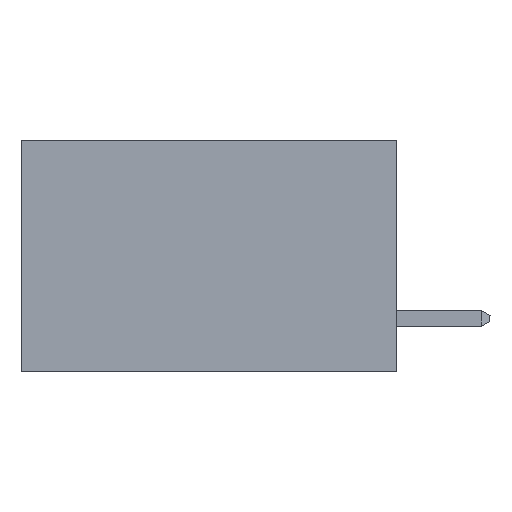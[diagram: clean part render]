
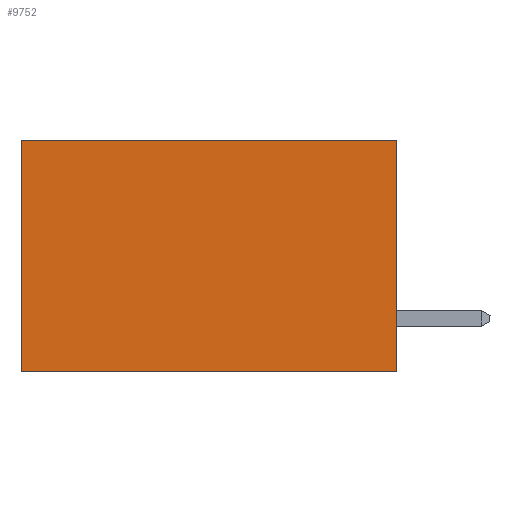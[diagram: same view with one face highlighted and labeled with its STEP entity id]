
A CAD part, left-side view. The second image highlights one B-rep face of the part: STEP entity #9752.
In plain terms, the highlighted planar face has unit normal (-1, 0, 0).
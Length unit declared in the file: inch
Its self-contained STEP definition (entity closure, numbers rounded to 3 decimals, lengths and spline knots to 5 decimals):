
#202 = VERTEX_POINT ( 'NONE', #7632 ) ;
#318 = EDGE_CURVE ( 'NONE', #1849, #520, #6760, .T. ) ;
#520 = VERTEX_POINT ( 'NONE', #635 ) ;
#635 = CARTESIAN_POINT ( 'NONE',  ( 0.2615, 0.6, -0.37 ) ) ;
#714 = DIRECTION ( 'NONE',  ( 1., 0., 0. ) ) ;
#820 = DIRECTION ( 'NONE',  ( 0., 0., -1. ) ) ;
#1398 = EDGE_CURVE ( 'NONE', #202, #8984, #6549, .T. ) ;
#1526 = DIRECTION ( 'NONE',  ( 0., 0., -1. ) ) ;
#1849 = VERTEX_POINT ( 'NONE', #8227 ) ;
#1892 = EDGE_CURVE ( 'NONE', #202, #1849, #9876, .T. ) ;
#2464 = ORIENTED_EDGE ( 'NONE', *, *, #1398, .T. ) ;
#3148 = LINE ( 'NONE', #3204, #3722 ) ;
#3166 = EDGE_CURVE ( 'NONE', #8984, #520, #3148, .T. ) ;
#3204 = CARTESIAN_POINT ( 'NONE',  ( 0.2615, 0.6, -0.37 ) ) ;
#3722 = VECTOR ( 'NONE', #8221, 39.37008 ) ;
#4135 = FACE_OUTER_BOUND ( 'NONE', #5857, .T. ) ;
#4335 = CARTESIAN_POINT ( 'NONE',  ( 0.2615, 0., -0.37 ) ) ;
#4891 = ORIENTED_EDGE ( 'NONE', *, *, #1892, .F. ) ;
#5191 = VECTOR ( 'NONE', #1526, 39.37008 ) ;
#5248 = CARTESIAN_POINT ( 'NONE',  ( 0.2615, 0.6, 0. ) ) ;
#5254 = DIRECTION ( 'NONE',  ( 0., 1., 0. ) ) ;
#5304 = VECTOR ( 'NONE', #9260, 39.37008 ) ;
#5447 = ORIENTED_EDGE ( 'NONE', *, *, #318, .F. ) ;
#5857 = EDGE_LOOP ( 'NONE', ( #10470, #5447, #4891, #2464 ) ) ;
#6549 = LINE ( 'NONE', #8293, #5304 ) ;
#6662 = CARTESIAN_POINT ( 'NONE',  ( 0.2615, 0., -0.37 ) ) ;
#6760 = LINE ( 'NONE', #4335, #9263 ) ;
#6941 = AXIS2_PLACEMENT_3D ( 'NONE', #6662, #714, #820 ) ;
#7486 = PLANE ( 'NONE',  #6941 ) ;
#7632 = CARTESIAN_POINT ( 'NONE',  ( 0.2615, 0., 0. ) ) ;
#8221 = DIRECTION ( 'NONE',  ( 0., 0., -1. ) ) ;
#8227 = CARTESIAN_POINT ( 'NONE',  ( 0.2615, 0., -0.37 ) ) ;
#8293 = CARTESIAN_POINT ( 'NONE',  ( 0.2615, 0., 0. ) ) ;
#8984 = VERTEX_POINT ( 'NONE', #5248 ) ;
#9139 = CARTESIAN_POINT ( 'NONE',  ( 0.2615, 0., -0.37 ) ) ;
#9260 = DIRECTION ( 'NONE',  ( 0., 1., 0. ) ) ;
#9263 = VECTOR ( 'NONE', #5254, 39.37008 ) ;
#9752 = ADVANCED_FACE ( 'NONE', ( #4135 ), #7486, .F. ) ;
#9876 = LINE ( 'NONE', #9139, #5191 ) ;
#10470 = ORIENTED_EDGE ( 'NONE', *, *, #3166, .T. ) ;
